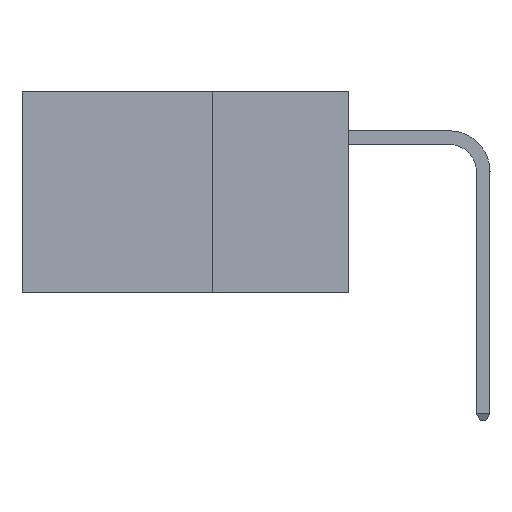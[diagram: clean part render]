
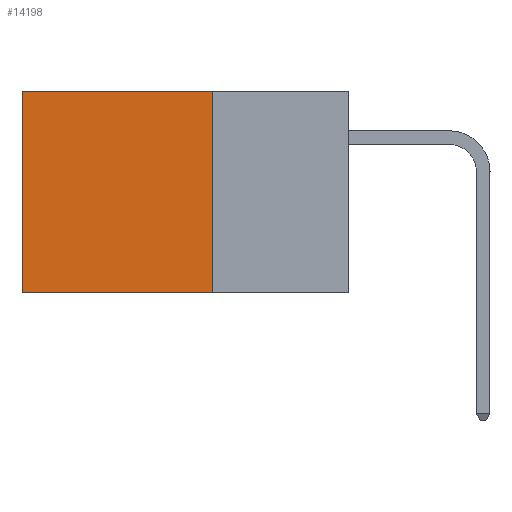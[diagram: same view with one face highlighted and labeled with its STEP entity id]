
A CAD part, left-side view. The second image highlights one B-rep face of the part: STEP entity #14198.
In plain terms, the highlighted planar face has unit normal (-1, 0, 0).
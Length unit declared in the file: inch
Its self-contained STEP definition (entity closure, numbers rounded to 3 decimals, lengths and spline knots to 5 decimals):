
#162 = DIRECTION ( 'NONE',  ( 0., 0., -1. ) ) ;
#612 = LINE ( 'NONE', #21860, #5337 ) ;
#791 = DIRECTION ( 'NONE',  ( 0., 1., 0. ) ) ;
#1521 = CARTESIAN_POINT ( 'NONE',  ( 0.2875, 0.25, 0. ) ) ;
#4684 = FACE_OUTER_BOUND ( 'NONE', #15904, .T. ) ;
#5337 = VECTOR ( 'NONE', #7073, 39.37008 ) ;
#6192 = ORIENTED_EDGE ( 'NONE', *, *, #23452, .T. ) ;
#7073 = DIRECTION ( 'NONE',  ( 0., 1., 0. ) ) ;
#9726 = ORIENTED_EDGE ( 'NONE', *, *, #39527, .T. ) ;
#10041 = ORIENTED_EDGE ( 'NONE', *, *, #44698, .F. ) ;
#10769 = LINE ( 'NONE', #31810, #42831 ) ;
#10996 = CARTESIAN_POINT ( 'NONE',  ( 0.2875, 0.25, 0. ) ) ;
#11094 = CARTESIAN_POINT ( 'NONE',  ( 0.2875, 0.25, -0.37 ) ) ;
#11176 = CARTESIAN_POINT ( 'NONE',  ( 0.2875, 0.25, -0.37 ) ) ;
#11684 = LINE ( 'NONE', #1521, #14264 ) ;
#12140 = DIRECTION ( 'NONE',  ( 0., 0., -1. ) ) ;
#13064 = CARTESIAN_POINT ( 'NONE',  ( 0.2875, 0.6, -0.37 ) ) ;
#14198 = ADVANCED_FACE ( 'NONE', ( #4684 ), #24879, .F. ) ;
#14264 = VECTOR ( 'NONE', #12140, 39.37008 ) ;
#15289 = VERTEX_POINT ( 'NONE', #43657 ) ;
#15904 = EDGE_LOOP ( 'NONE', ( #9726, #29234, #10041, #6192 ) ) ;
#16703 = VERTEX_POINT ( 'NONE', #21394 ) ;
#20201 = VECTOR ( 'NONE', #791, 39.37008 ) ;
#21394 = CARTESIAN_POINT ( 'NONE',  ( 0.2875, 0.6, 0. ) ) ;
#21852 = DIRECTION ( 'NONE',  ( 0., 0., -1. ) ) ;
#21860 = CARTESIAN_POINT ( 'NONE',  ( 0.2875, 0.25, 0. ) ) ;
#23452 = EDGE_CURVE ( 'NONE', #15289, #16703, #612, .T. ) ;
#24650 = DIRECTION ( 'NONE',  ( 1., 0., 0. ) ) ;
#24879 = PLANE ( 'NONE',  #38919 ) ;
#29234 = ORIENTED_EDGE ( 'NONE', *, *, #45014, .F. ) ;
#31281 = VERTEX_POINT ( 'NONE', #11094 ) ;
#31810 = CARTESIAN_POINT ( 'NONE',  ( 0.2875, 0.6, 0. ) ) ;
#32455 = LINE ( 'NONE', #11176, #20201 ) ;
#38919 = AXIS2_PLACEMENT_3D ( 'NONE', #10996, #24650, #162 ) ;
#39527 = EDGE_CURVE ( 'NONE', #16703, #43617, #10769, .T. ) ;
#42831 = VECTOR ( 'NONE', #21852, 39.37008 ) ;
#43617 = VERTEX_POINT ( 'NONE', #13064 ) ;
#43657 = CARTESIAN_POINT ( 'NONE',  ( 0.2875, 0.25, 0. ) ) ;
#44698 = EDGE_CURVE ( 'NONE', #15289, #31281, #11684, .T. ) ;
#45014 = EDGE_CURVE ( 'NONE', #31281, #43617, #32455, .T. ) ;
